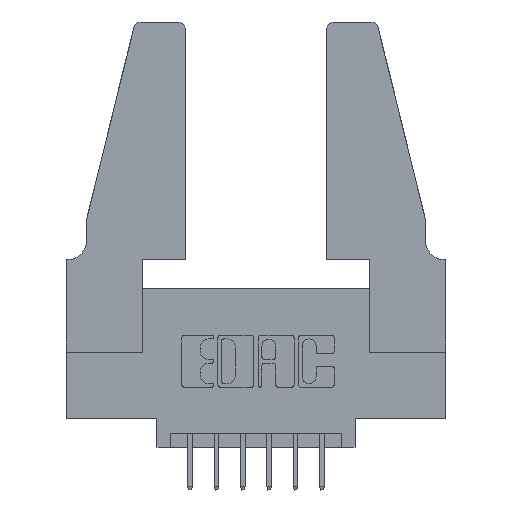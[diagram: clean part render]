
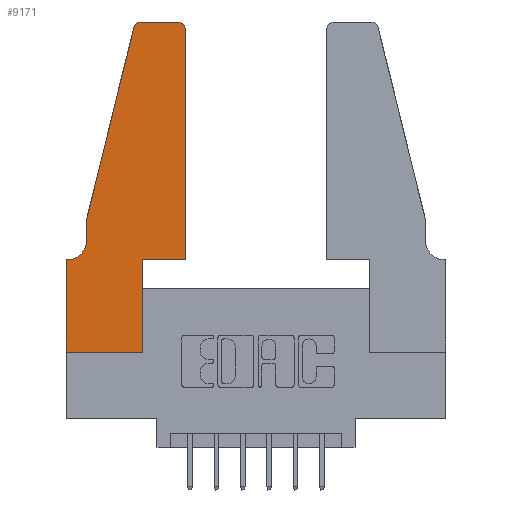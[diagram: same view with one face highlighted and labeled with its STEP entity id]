
A CAD part, top view. The second image highlights one B-rep face of the part: STEP entity #9171.
In plain terms, the highlighted planar face has unit normal (0, 0, 1).
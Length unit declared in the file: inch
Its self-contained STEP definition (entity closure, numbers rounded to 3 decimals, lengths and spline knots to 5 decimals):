
#56 = ORIENTED_EDGE ( 'NONE', *, *, #7648, .T. ) ;
#87 = CARTESIAN_POINT ( 'NONE',  ( 0.284, 1.25, 0.37 ) ) ;
#159 = LINE ( 'NONE', #539, #9195 ) ;
#217 = CARTESIAN_POINT ( 'NONE',  ( 0.0755, 0.35, 0.37 ) ) ;
#225 = CARTESIAN_POINT ( 'NONE',  ( 0.2865, 0.35, 0.37 ) ) ;
#240 = DIRECTION ( 'NONE',  ( 1., 0., 0. ) ) ;
#324 = DIRECTION ( 'NONE',  ( 0., 0., 1. ) ) ;
#329 = EDGE_CURVE ( 'NONE', #11758, #8632, #6336, .T. ) ;
#405 = VERTEX_POINT ( 'NONE', #7051 ) ;
#449 = EDGE_CURVE ( 'NONE', #3413, #11631, #159, .T. ) ;
#539 = CARTESIAN_POINT ( 'NONE',  ( 0.4505, 0.35, 0.37 ) ) ;
#604 = CARTESIAN_POINT ( 'NONE',  ( 0.0055, 0.35, 0.37 ) ) ;
#674 = LINE ( 'NONE', #8294, #972 ) ;
#972 = VECTOR ( 'NONE', #3606, 39.37008 ) ;
#1046 = DIRECTION ( 'NONE',  ( 0., 0., 1. ) ) ;
#1164 = LINE ( 'NONE', #11487, #7910 ) ;
#1208 = CARTESIAN_POINT ( 'NONE',  ( 0.25487, 1.22718, 0.37 ) ) ;
#1294 = FACE_OUTER_BOUND ( 'NONE', #11186, .T. ) ;
#1399 = DIRECTION ( 'NONE',  ( 0., -1., 0. ) ) ;
#1446 = ORIENTED_EDGE ( 'NONE', *, *, #10580, .T. ) ;
#1494 = DIRECTION ( 'NONE',  ( 1., 0., 0. ) ) ;
#1651 = DIRECTION ( 'NONE',  ( 1., 0., 0. ) ) ;
#1829 = CARTESIAN_POINT ( 'NONE',  ( 0.2865, 0.35, 0.37 ) ) ;
#1905 = VERTEX_POINT ( 'NONE', #9269 ) ;
#1961 = ORIENTED_EDGE ( 'NONE', *, *, #10700, .T. ) ;
#2026 = CARTESIAN_POINT ( 'NONE',  ( 0.4205, 1.22, 0.37 ) ) ;
#2033 = LINE ( 'NONE', #4344, #11859 ) ;
#2225 = AXIS2_PLACEMENT_3D ( 'NONE', #2026, #1046, #11302 ) ;
#2444 = CARTESIAN_POINT ( 'NONE',  ( 0.0055, 0.42, 0.37 ) ) ;
#2722 = LINE ( 'NONE', #217, #8877 ) ;
#2873 = EDGE_CURVE ( 'NONE', #9515, #11758, #1164, .T. ) ;
#3262 = PLANE ( 'NONE',  #7975 ) ;
#3413 = VERTEX_POINT ( 'NONE', #5919 ) ;
#3606 = DIRECTION ( 'NONE',  ( 0., -1., 0. ) ) ;
#3809 = LINE ( 'NONE', #225, #9098 ) ;
#3832 = ORIENTED_EDGE ( 'NONE', *, *, #11782, .T. ) ;
#3922 = DIRECTION ( 'NONE',  ( 0., 1., 0. ) ) ;
#4040 = VERTEX_POINT ( 'NONE', #6724 ) ;
#4114 = LINE ( 'NONE', #7954, #5984 ) ;
#4197 = DIRECTION ( 'NONE',  ( 0., 0., -1. ) ) ;
#4316 = DIRECTION ( 'NONE',  ( 0., 1., 0. ) ) ;
#4344 = CARTESIAN_POINT ( 'NONE',  ( 0.0755, 0.5, 0.37 ) ) ;
#4477 = VERTEX_POINT ( 'NONE', #87 ) ;
#4769 = EDGE_CURVE ( 'NONE', #8632, #405, #2722, .T. ) ;
#5101 = ORIENTED_EDGE ( 'NONE', *, *, #11838, .T. ) ;
#5182 = ORIENTED_EDGE ( 'NONE', *, *, #449, .T. ) ;
#5378 = ORIENTED_EDGE ( 'NONE', *, *, #2873, .T. ) ;
#5612 = ORIENTED_EDGE ( 'NONE', *, *, #329, .T. ) ;
#5718 = CIRCLE ( 'NONE', #2225, 0.03 ) ;
#5726 = DIRECTION ( 'NONE',  ( -1., 0., 0. ) ) ;
#5919 = CARTESIAN_POINT ( 'NONE',  ( 0.4505, 0.35, 0.37 ) ) ;
#5982 = CARTESIAN_POINT ( 'NONE',  ( 0., 0.35, 0.37 ) ) ;
#5984 = VECTOR ( 'NONE', #1494, 39.37008 ) ;
#6081 = DIRECTION ( 'NONE',  ( 1., 0., 0. ) ) ;
#6174 = DIRECTION ( 'NONE',  ( -1., 0., 0. ) ) ;
#6336 = CIRCLE ( 'NONE', #10135, 0.07 ) ;
#6724 = CARTESIAN_POINT ( 'NONE',  ( 0., 0., 0.37 ) ) ;
#6887 = AXIS2_PLACEMENT_3D ( 'NONE', #11246, #324, #240 ) ;
#6925 = EDGE_CURVE ( 'NONE', #4477, #9064, #9245, .T. ) ;
#7051 = CARTESIAN_POINT ( 'NONE',  ( 0., 0.35, 0.37 ) ) ;
#7113 = EDGE_CURVE ( 'NONE', #9430, #10510, #3809, .T. ) ;
#7206 = ORIENTED_EDGE ( 'NONE', *, *, #4769, .T. ) ;
#7630 = EDGE_CURVE ( 'NONE', #9064, #9515, #2033, .T. ) ;
#7648 = EDGE_CURVE ( 'NONE', #1905, #4477, #9534, .T. ) ;
#7910 = VECTOR ( 'NONE', #1399, 39.37008 ) ;
#7954 = CARTESIAN_POINT ( 'NONE',  ( 0.4505, 0.35, 0.37 ) ) ;
#7975 = AXIS2_PLACEMENT_3D ( 'NONE', #5982, #9742, #6081 ) ;
#8294 = CARTESIAN_POINT ( 'NONE',  ( 0., 0., 0.37 ) ) ;
#8515 = CARTESIAN_POINT ( 'NONE',  ( 0.2865, 0., 0.37 ) ) ;
#8632 = VERTEX_POINT ( 'NONE', #604 ) ;
#8672 = CARTESIAN_POINT ( 'NONE',  ( 0.4505, 1.22, 0.37 ) ) ;
#8795 = VECTOR ( 'NONE', #6174, 39.37008 ) ;
#8877 = VECTOR ( 'NONE', #5726, 39.37008 ) ;
#9064 = VERTEX_POINT ( 'NONE', #1208 ) ;
#9098 = VECTOR ( 'NONE', #3922, 39.37008 ) ;
#9171 = ADVANCED_FACE ( 'NONE', ( #1294 ), #3262, .T. ) ;
#9195 = VECTOR ( 'NONE', #4316, 39.37008 ) ;
#9245 = CIRCLE ( 'NONE', #6887, 0.03 ) ;
#9269 = CARTESIAN_POINT ( 'NONE',  ( 0.4205, 1.25, 0.37 ) ) ;
#9430 = VERTEX_POINT ( 'NONE', #8515 ) ;
#9515 = VERTEX_POINT ( 'NONE', #10797 ) ;
#9534 = LINE ( 'NONE', #10732, #8795 ) ;
#9651 = DIRECTION ( 'NONE',  ( -1., 0., 0. ) ) ;
#9673 = ORIENTED_EDGE ( 'NONE', *, *, #7630, .T. ) ;
#9702 = VECTOR ( 'NONE', #1651, 39.37008 ) ;
#9742 = DIRECTION ( 'NONE',  ( 0., 0., 1. ) ) ;
#9862 = LINE ( 'NONE', #9912, #9702 ) ;
#9865 = ORIENTED_EDGE ( 'NONE', *, *, #7113, .T. ) ;
#9866 = CARTESIAN_POINT ( 'NONE',  ( 0.0755, 0.42, 0.37 ) ) ;
#9912 = CARTESIAN_POINT ( 'NONE',  ( 0., 0., 0.37 ) ) ;
#10135 = AXIS2_PLACEMENT_3D ( 'NONE', #2444, #4197, #9651 ) ;
#10510 = VERTEX_POINT ( 'NONE', #1829 ) ;
#10580 = EDGE_CURVE ( 'NONE', #405, #4040, #674, .T. ) ;
#10700 = EDGE_CURVE ( 'NONE', #11631, #1905, #5718, .T. ) ;
#10732 = CARTESIAN_POINT ( 'NONE',  ( 0.2605, 1.25, 0.37 ) ) ;
#10797 = CARTESIAN_POINT ( 'NONE',  ( 0.0755, 0.5, 0.37 ) ) ;
#10874 = DIRECTION ( 'NONE',  ( -0.239, -0.971, 0. ) ) ;
#10937 = ORIENTED_EDGE ( 'NONE', *, *, #6925, .T. ) ;
#11186 = EDGE_LOOP ( 'NONE', ( #56, #10937, #9673, #5378, #5612, #7206, #1446, #5101, #9865, #3832, #5182, #1961 ) ) ;
#11246 = CARTESIAN_POINT ( 'NONE',  ( 0.284, 1.22, 0.37 ) ) ;
#11302 = DIRECTION ( 'NONE',  ( 1., 0., 0. ) ) ;
#11487 = CARTESIAN_POINT ( 'NONE',  ( 0.0755, 0.5, 0.37 ) ) ;
#11631 = VERTEX_POINT ( 'NONE', #8672 ) ;
#11758 = VERTEX_POINT ( 'NONE', #9866 ) ;
#11782 = EDGE_CURVE ( 'NONE', #10510, #3413, #4114, .T. ) ;
#11838 = EDGE_CURVE ( 'NONE', #4040, #9430, #9862, .T. ) ;
#11859 = VECTOR ( 'NONE', #10874, 39.37008 ) ;
